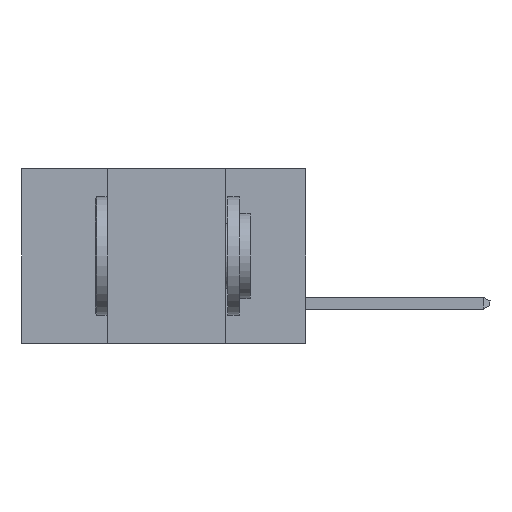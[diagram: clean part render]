
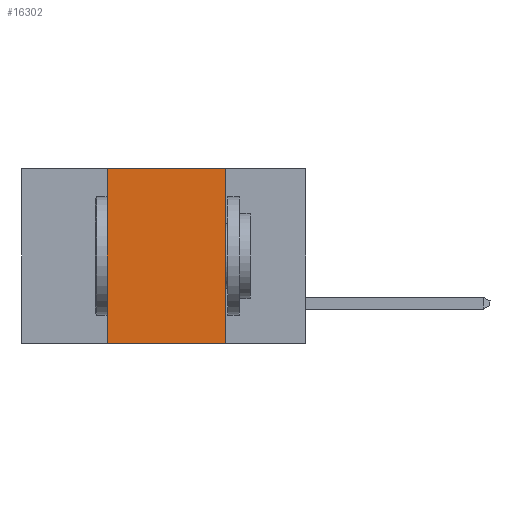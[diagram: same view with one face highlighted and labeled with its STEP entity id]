
A CAD part, left-side view. The second image highlights one B-rep face of the part: STEP entity #16302.
In plain terms, the highlighted planar face has unit normal (-1, 0, 0).
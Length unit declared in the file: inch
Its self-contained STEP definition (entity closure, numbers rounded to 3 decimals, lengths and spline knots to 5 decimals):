
#385 = DIRECTION ( 'NONE',  ( 0., 0., -1. ) ) ;
#785 = VECTOR ( 'NONE', #9279, 39.37008 ) ;
#1031 = CARTESIAN_POINT ( 'NONE',  ( 0., 0.6, -0.37 ) ) ;
#2579 = FACE_OUTER_BOUND ( 'NONE', #6179, .T. ) ;
#2751 = DIRECTION ( 'NONE',  ( 0., 0., -1. ) ) ;
#2883 = CARTESIAN_POINT ( 'NONE',  ( 0., 0.17, -0.37 ) ) ;
#3568 = CARTESIAN_POINT ( 'NONE',  ( 0., 0.17, -0.37 ) ) ;
#6118 = VERTEX_POINT ( 'NONE', #7449 ) ;
#6179 = EDGE_LOOP ( 'NONE', ( #23281, #12270, #12281, #15713 ) ) ;
#6579 = LINE ( 'NONE', #2883, #6770 ) ;
#6770 = VECTOR ( 'NONE', #2751, 39.37008 ) ;
#6811 = CARTESIAN_POINT ( 'NONE',  ( 0., 0.6, 0. ) ) ;
#7449 = CARTESIAN_POINT ( 'NONE',  ( 0., 0.42, 0. ) ) ;
#9133 = CARTESIAN_POINT ( 'NONE',  ( 0., 0.17, 0. ) ) ;
#9279 = DIRECTION ( 'NONE',  ( 0., 0., 1. ) ) ;
#10082 = EDGE_CURVE ( 'NONE', #14460, #6118, #12412, .T. ) ;
#10391 = VECTOR ( 'NONE', #19614, 39.37008 ) ;
#12270 = ORIENTED_EDGE ( 'NONE', *, *, #26037, .F. ) ;
#12281 = ORIENTED_EDGE ( 'NONE', *, *, #10082, .F. ) ;
#12412 = LINE ( 'NONE', #24837, #785 ) ;
#13999 = VECTOR ( 'NONE', #18735, 39.37008 ) ;
#14460 = VERTEX_POINT ( 'NONE', #20489 ) ;
#14566 = VERTEX_POINT ( 'NONE', #9133 ) ;
#14911 = CARTESIAN_POINT ( 'NONE',  ( 0., 0.6, 0. ) ) ;
#15713 = ORIENTED_EDGE ( 'NONE', *, *, #22694, .T. ) ;
#16302 = ADVANCED_FACE ( 'NONE', ( #2579 ), #25497, .F. ) ;
#17154 = EDGE_CURVE ( 'NONE', #14566, #17276, #6579, .T. ) ;
#17183 = AXIS2_PLACEMENT_3D ( 'NONE', #6811, #19098, #385 ) ;
#17276 = VERTEX_POINT ( 'NONE', #3568 ) ;
#18735 = DIRECTION ( 'NONE',  ( 0., -1., 0. ) ) ;
#19098 = DIRECTION ( 'NONE',  ( 1., 0., 0. ) ) ;
#19614 = DIRECTION ( 'NONE',  ( 0., -1., 0. ) ) ;
#20489 = CARTESIAN_POINT ( 'NONE',  ( 0., 0.42, -0.37 ) ) ;
#22694 = EDGE_CURVE ( 'NONE', #14460, #17276, #25749, .T. ) ;
#23281 = ORIENTED_EDGE ( 'NONE', *, *, #17154, .F. ) ;
#24837 = CARTESIAN_POINT ( 'NONE',  ( 0., 0.42, -0.37 ) ) ;
#25497 = PLANE ( 'NONE',  #17183 ) ;
#25749 = LINE ( 'NONE', #1031, #10391 ) ;
#26037 = EDGE_CURVE ( 'NONE', #6118, #14566, #26917, .T. ) ;
#26917 = LINE ( 'NONE', #14911, #13999 ) ;
